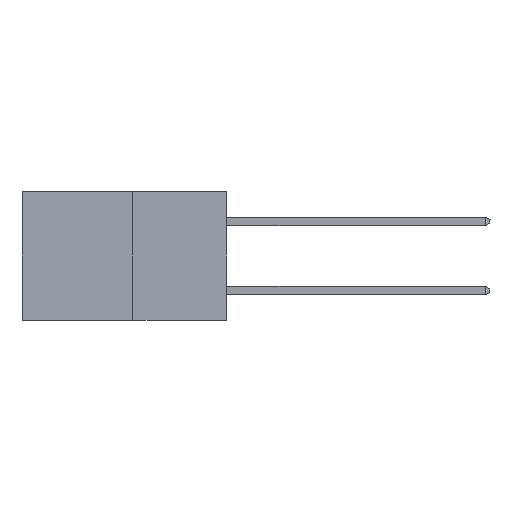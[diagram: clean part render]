
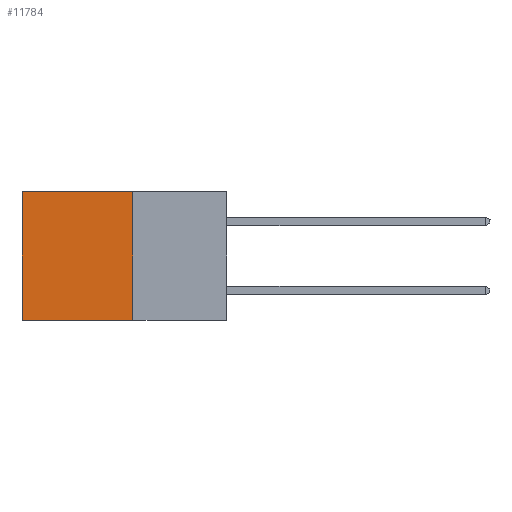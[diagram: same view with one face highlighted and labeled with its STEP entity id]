
A CAD part, left-side view. The second image highlights one B-rep face of the part: STEP entity #11784.
In plain terms, the highlighted planar face has unit normal (-1, 0, 0).
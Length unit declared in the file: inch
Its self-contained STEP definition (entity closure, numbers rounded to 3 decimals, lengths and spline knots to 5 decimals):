
#31 = DIRECTION ( 'NONE',  ( 0., 0., -1. ) ) ;
#99 = FACE_OUTER_BOUND ( 'NONE', #10247, .T. ) ;
#1662 = ORIENTED_EDGE ( 'NONE', *, *, #16370, .T. ) ;
#1874 = ORIENTED_EDGE ( 'NONE', *, *, #14868, .F. ) ;
#2349 = LINE ( 'NONE', #11612, #13430 ) ;
#3188 = LINE ( 'NONE', #10903, #10455 ) ;
#4018 = AXIS2_PLACEMENT_3D ( 'NONE', #13857, #15320, #6835 ) ;
#4313 = ORIENTED_EDGE ( 'NONE', *, *, #7816, .F. ) ;
#4732 = VERTEX_POINT ( 'NONE', #7354 ) ;
#5836 = VECTOR ( 'NONE', #10052, 39.37008 ) ;
#5894 = VECTOR ( 'NONE', #9783, 39.37008 ) ;
#6835 = DIRECTION ( 'NONE',  ( 0., 0., -1. ) ) ;
#6849 = ORIENTED_EDGE ( 'NONE', *, *, #13346, .T. ) ;
#7354 = CARTESIAN_POINT ( 'NONE',  ( 0.277, 0.59, -0.37 ) ) ;
#7816 = EDGE_CURVE ( 'NONE', #15592, #10791, #3188, .T. ) ;
#8716 = CARTESIAN_POINT ( 'NONE',  ( 0.277, 0.27, 0. ) ) ;
#9783 = DIRECTION ( 'NONE',  ( 0., 1., 0. ) ) ;
#10052 = DIRECTION ( 'NONE',  ( 0., 1., 0. ) ) ;
#10247 = EDGE_LOOP ( 'NONE', ( #1662, #1874, #4313, #6849 ) ) ;
#10442 = DIRECTION ( 'NONE',  ( 0., 0., -1. ) ) ;
#10455 = VECTOR ( 'NONE', #10442, 39.37008 ) ;
#10791 = VERTEX_POINT ( 'NONE', #15720 ) ;
#10903 = CARTESIAN_POINT ( 'NONE',  ( 0.277, 0.27, -0.37 ) ) ;
#11612 = CARTESIAN_POINT ( 'NONE',  ( 0.277, 0.59, -0.37 ) ) ;
#11784 = ADVANCED_FACE ( 'NONE', ( #99 ), #16635, .F. ) ;
#12528 = LINE ( 'NONE', #8716, #5836 ) ;
#13346 = EDGE_CURVE ( 'NONE', #15592, #15528, #12528, .T. ) ;
#13430 = VECTOR ( 'NONE', #31, 39.37008 ) ;
#13857 = CARTESIAN_POINT ( 'NONE',  ( 0.277, 0.27, -0.37 ) ) ;
#14233 = CARTESIAN_POINT ( 'NONE',  ( 0.277, 0.27, 0. ) ) ;
#14868 = EDGE_CURVE ( 'NONE', #10791, #4732, #16773, .T. ) ;
#15320 = DIRECTION ( 'NONE',  ( 1., 0., 0. ) ) ;
#15528 = VERTEX_POINT ( 'NONE', #16910 ) ;
#15592 = VERTEX_POINT ( 'NONE', #14233 ) ;
#15720 = CARTESIAN_POINT ( 'NONE',  ( 0.277, 0.27, -0.37 ) ) ;
#16370 = EDGE_CURVE ( 'NONE', #15528, #4732, #2349, .T. ) ;
#16635 = PLANE ( 'NONE',  #4018 ) ;
#16773 = LINE ( 'NONE', #18160, #5894 ) ;
#16910 = CARTESIAN_POINT ( 'NONE',  ( 0.277, 0.59, 0. ) ) ;
#18160 = CARTESIAN_POINT ( 'NONE',  ( 0.277, 0.27, -0.37 ) ) ;
